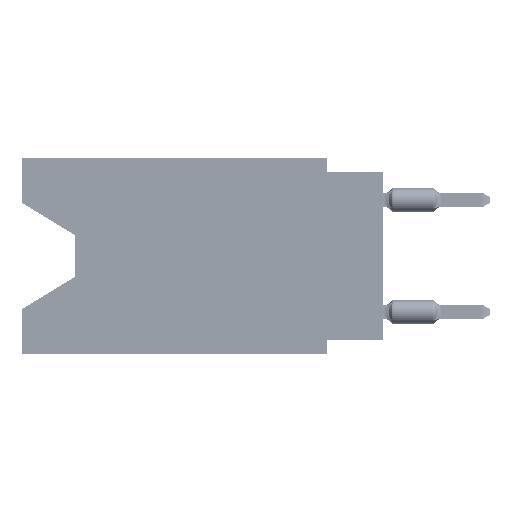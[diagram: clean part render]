
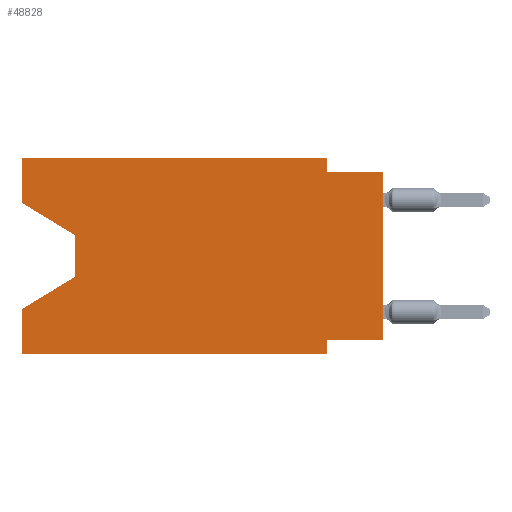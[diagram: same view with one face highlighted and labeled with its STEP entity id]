
A CAD part, left-side view. The second image highlights one B-rep face of the part: STEP entity #48828.
In plain terms, the highlighted planar face has unit normal (-1, 0, 0).
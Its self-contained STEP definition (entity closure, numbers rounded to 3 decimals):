
#1907 = DIRECTION ( 'NONE',  ( 0., -0.855, -0.519 ) ) ;
#3814 = FACE_OUTER_BOUND ( 'NONE', #19110, .T. ) ;
#3931 = EDGE_CURVE ( 'NONE', #21285, #57293, #18682, .T. ) ;
#4167 = ORIENTED_EDGE ( 'NONE', *, *, #33162, .T. ) ;
#4759 = VERTEX_POINT ( 'NONE', #27902 ) ;
#5345 = CARTESIAN_POINT ( 'NONE',  ( 0., 13.97, -5.385 ) ) ;
#6379 = DIRECTION ( 'NONE',  ( 0., 0., -1. ) ) ;
#6425 = ORIENTED_EDGE ( 'NONE', *, *, #61372, .T. ) ;
#6444 = ORIENTED_EDGE ( 'NONE', *, *, #37374, .F. ) ;
#7363 = LINE ( 'NONE', #44375, #43550 ) ;
#7447 = CARTESIAN_POINT ( 'NONE',  ( 0., 16.383, -8.89 ) ) ;
#8219 = LINE ( 'NONE', #13241, #9456 ) ;
#9320 = LINE ( 'NONE', #65493, #16215 ) ;
#9456 = VECTOR ( 'NONE', #1907, 1000. ) ;
#9915 = DIRECTION ( 'NONE',  ( 0., 0., 1. ) ) ;
#11482 = ORIENTED_EDGE ( 'NONE', *, *, #26515, .F. ) ;
#13241 = CARTESIAN_POINT ( 'NONE',  ( 0., 16.383, -2.038 ) ) ;
#14861 = PLANE ( 'NONE',  #42910 ) ;
#15138 = CARTESIAN_POINT ( 'NONE',  ( 0., 0., -0.635 ) ) ;
#15518 = DIRECTION ( 'NONE',  ( 0., 0., 1. ) ) ;
#16215 = VECTOR ( 'NONE', #56460, 1000. ) ;
#17093 = LINE ( 'NONE', #42494, #58592 ) ;
#18682 = LINE ( 'NONE', #42763, #56776 ) ;
#19110 = EDGE_LOOP ( 'NONE', ( #39382, #61256, #6425, #51787, #24735, #29511, #19116, #4167, #11482, #58429, #6444, #25029 ) ) ;
#19116 = ORIENTED_EDGE ( 'NONE', *, *, #27559, .F. ) ;
#21285 = VERTEX_POINT ( 'NONE', #7447 ) ;
#23235 = VECTOR ( 'NONE', #30085, 1000. ) ;
#24735 = ORIENTED_EDGE ( 'NONE', *, *, #55719, .T. ) ;
#25029 = ORIENTED_EDGE ( 'NONE', *, *, #33783, .F. ) ;
#25257 = VECTOR ( 'NONE', #9915, 1000. ) ;
#25335 = CARTESIAN_POINT ( 'NONE',  ( 0., 16.383, 0. ) ) ;
#26283 = VECTOR ( 'NONE', #52494, 1000. ) ;
#26464 = CARTESIAN_POINT ( 'NONE',  ( 0., 13.97, -3.505 ) ) ;
#26468 = EDGE_CURVE ( 'NONE', #55692, #32373, #7363, .T. ) ;
#26515 = EDGE_CURVE ( 'NONE', #43379, #41110, #50077, .T. ) ;
#26924 = VECTOR ( 'NONE', #52775, 1000. ) ;
#27097 = VERTEX_POINT ( 'NONE', #31247 ) ;
#27559 = EDGE_CURVE ( 'NONE', #27097, #65097, #60502, .T. ) ;
#27646 = CARTESIAN_POINT ( 'NONE',  ( 0., 2.54, -0.635 ) ) ;
#27902 = CARTESIAN_POINT ( 'NONE',  ( 0., 2.54, -8.89 ) ) ;
#29511 = ORIENTED_EDGE ( 'NONE', *, *, #30498, .F. ) ;
#30085 = DIRECTION ( 'NONE',  ( 0., 1., 0. ) ) ;
#30235 = VERTEX_POINT ( 'NONE', #38864 ) ;
#30498 = EDGE_CURVE ( 'NONE', #65097, #4759, #17093, .T. ) ;
#31247 = CARTESIAN_POINT ( 'NONE',  ( 0., 0., -8.255 ) ) ;
#32373 = VERTEX_POINT ( 'NONE', #55884 ) ;
#32637 = VECTOR ( 'NONE', #15518, 1000. ) ;
#33162 = EDGE_CURVE ( 'NONE', #27097, #41110, #56313, .T. ) ;
#33783 = EDGE_CURVE ( 'NONE', #51712, #59409, #66111, .T. ) ;
#34357 = DIRECTION ( 'NONE',  ( 0., 0., -1. ) ) ;
#37084 = LINE ( 'NONE', #5345, #26924 ) ;
#37134 = CARTESIAN_POINT ( 'NONE',  ( 0., 16.383, -8.89 ) ) ;
#37374 = EDGE_CURVE ( 'NONE', #59409, #30235, #63478, .T. ) ;
#38864 = CARTESIAN_POINT ( 'NONE',  ( 0., 2.54, 0. ) ) ;
#39382 = ORIENTED_EDGE ( 'NONE', *, *, #39464, .T. ) ;
#39464 = EDGE_CURVE ( 'NONE', #51712, #55692, #8219, .T. ) ;
#41110 = VERTEX_POINT ( 'NONE', #15138 ) ;
#41529 = VECTOR ( 'NONE', #45048, 1000. ) ;
#42307 = VECTOR ( 'NONE', #43412, 1000. ) ;
#42494 = CARTESIAN_POINT ( 'NONE',  ( 0., 2.54, -8.89 ) ) ;
#42763 = CARTESIAN_POINT ( 'NONE',  ( 0., 16.383, 0. ) ) ;
#42910 = AXIS2_PLACEMENT_3D ( 'NONE', #55647, #59995, #59671 ) ;
#43379 = VERTEX_POINT ( 'NONE', #27646 ) ;
#43412 = DIRECTION ( 'NONE',  ( 0., -1., 0. ) ) ;
#43550 = VECTOR ( 'NONE', #34357, 1000. ) ;
#44375 = CARTESIAN_POINT ( 'NONE',  ( 0., 13.97, -3.505 ) ) ;
#45048 = DIRECTION ( 'NONE',  ( 0., -1., 0. ) ) ;
#45103 = CARTESIAN_POINT ( 'NONE',  ( 0., 16.383, -2.038 ) ) ;
#47347 = CARTESIAN_POINT ( 'NONE',  ( 0., 16.383, -6.852 ) ) ;
#48138 = DIRECTION ( 'NONE',  ( 0., 0., 1. ) ) ;
#48828 = ADVANCED_FACE ( 'NONE', ( #3814 ), #14861, .F. ) ;
#50077 = LINE ( 'NONE', #63540, #41529 ) ;
#50918 = CARTESIAN_POINT ( 'NONE',  ( 0., 16.383, 0. ) ) ;
#51712 = VERTEX_POINT ( 'NONE', #45103 ) ;
#51787 = ORIENTED_EDGE ( 'NONE', *, *, #3931, .F. ) ;
#52494 = DIRECTION ( 'NONE',  ( 0., -1., 0. ) ) ;
#52775 = DIRECTION ( 'NONE',  ( 0., 0.855, -0.519 ) ) ;
#53780 = CARTESIAN_POINT ( 'NONE',  ( 0., 16.383, 0. ) ) ;
#54825 = EDGE_CURVE ( 'NONE', #30235, #43379, #9320, .T. ) ;
#55647 = CARTESIAN_POINT ( 'NONE',  ( 0., 16.383, 0. ) ) ;
#55692 = VERTEX_POINT ( 'NONE', #26464 ) ;
#55719 = EDGE_CURVE ( 'NONE', #21285, #4759, #57217, .T. ) ;
#55884 = CARTESIAN_POINT ( 'NONE',  ( 0., 13.97, -5.385 ) ) ;
#56313 = LINE ( 'NONE', #66015, #32637 ) ;
#56460 = DIRECTION ( 'NONE',  ( 0., 0., -1. ) ) ;
#56776 = VECTOR ( 'NONE', #48138, 1000. ) ;
#57217 = LINE ( 'NONE', #37134, #26283 ) ;
#57293 = VERTEX_POINT ( 'NONE', #47347 ) ;
#58429 = ORIENTED_EDGE ( 'NONE', *, *, #54825, .F. ) ;
#58592 = VECTOR ( 'NONE', #6379, 1000. ) ;
#59409 = VERTEX_POINT ( 'NONE', #50918 ) ;
#59671 = DIRECTION ( 'NONE',  ( 0., 0., -1. ) ) ;
#59995 = DIRECTION ( 'NONE',  ( 1., 0., 0. ) ) ;
#60502 = LINE ( 'NONE', #60841, #23235 ) ;
#60841 = CARTESIAN_POINT ( 'NONE',  ( 0., 0., -8.255 ) ) ;
#61256 = ORIENTED_EDGE ( 'NONE', *, *, #26468, .T. ) ;
#61372 = EDGE_CURVE ( 'NONE', #32373, #57293, #37084, .T. ) ;
#63478 = LINE ( 'NONE', #53780, #42307 ) ;
#63540 = CARTESIAN_POINT ( 'NONE',  ( 0., 0., -0.635 ) ) ;
#64813 = CARTESIAN_POINT ( 'NONE',  ( 0., 2.54, -8.255 ) ) ;
#65097 = VERTEX_POINT ( 'NONE', #64813 ) ;
#65493 = CARTESIAN_POINT ( 'NONE',  ( 0., 2.54, 0. ) ) ;
#66015 = CARTESIAN_POINT ( 'NONE',  ( 0., 0., 0. ) ) ;
#66111 = LINE ( 'NONE', #25335, #25257 ) ;
